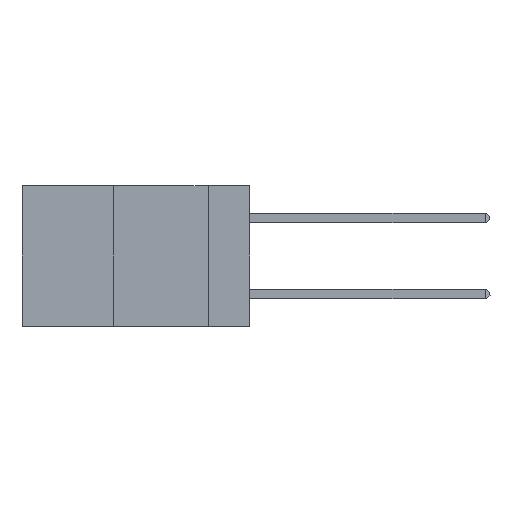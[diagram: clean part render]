
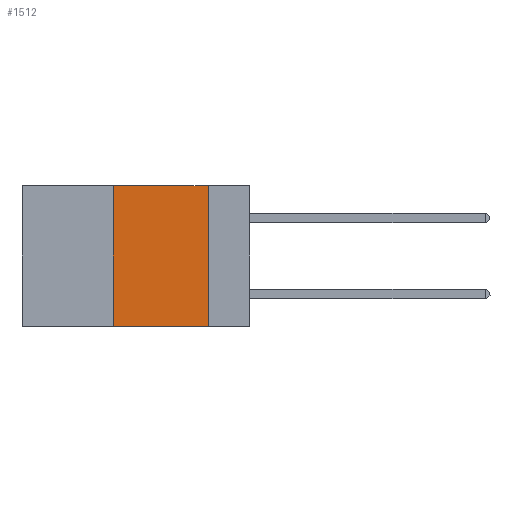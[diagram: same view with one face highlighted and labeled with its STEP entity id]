
A CAD part, left-side view. The second image highlights one B-rep face of the part: STEP entity #1512.
In plain terms, the highlighted planar face has unit normal (-1, 0, 0).
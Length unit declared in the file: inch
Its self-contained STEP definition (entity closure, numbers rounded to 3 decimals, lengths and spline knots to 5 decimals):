
#875 = VERTEX_POINT ( 'NONE', #9442 ) ;
#1187 = VECTOR ( 'NONE', #8809, 39.37008 ) ;
#1382 = PLANE ( 'NONE',  #9355 ) ;
#1512 = ADVANCED_FACE ( 'NONE', ( #8071 ), #1382, .F. ) ;
#1883 = VERTEX_POINT ( 'NONE', #3095 ) ;
#1942 = ORIENTED_EDGE ( 'NONE', *, *, #6858, .T. ) ;
#2199 = EDGE_LOOP ( 'NONE', ( #8537, #2297, #2607, #1942 ) ) ;
#2297 = ORIENTED_EDGE ( 'NONE', *, *, #10416, .F. ) ;
#2519 = CARTESIAN_POINT ( 'NONE',  ( 0., 0.11, 0. ) ) ;
#2555 = DIRECTION ( 'NONE',  ( 0., -1., 0. ) ) ;
#2586 = LINE ( 'NONE', #2689, #8052 ) ;
#2607 = ORIENTED_EDGE ( 'NONE', *, *, #7558, .F. ) ;
#2645 = CARTESIAN_POINT ( 'NONE',  ( 0., 0.11, 0. ) ) ;
#2689 = CARTESIAN_POINT ( 'NONE',  ( 0., 0.36, 0. ) ) ;
#3023 = DIRECTION ( 'NONE',  ( 0., 0., 1. ) ) ;
#3095 = CARTESIAN_POINT ( 'NONE',  ( 0., 0.36, 0. ) ) ;
#3147 = CARTESIAN_POINT ( 'NONE',  ( 0., 0.6, 0. ) ) ;
#4251 = VECTOR ( 'NONE', #7780, 39.37008 ) ;
#4694 = VECTOR ( 'NONE', #2555, 39.37008 ) ;
#5821 = DIRECTION ( 'NONE',  ( 0., 0., -1. ) ) ;
#5934 = DIRECTION ( 'NONE',  ( 1., 0., 0. ) ) ;
#6052 = VERTEX_POINT ( 'NONE', #2645 ) ;
#6630 = LINE ( 'NONE', #6940, #4251 ) ;
#6641 = LINE ( 'NONE', #8933, #4694 ) ;
#6803 = EDGE_CURVE ( 'NONE', #6052, #11433, #7208, .T. ) ;
#6858 = EDGE_CURVE ( 'NONE', #875, #11433, #6641, .T. ) ;
#6940 = CARTESIAN_POINT ( 'NONE',  ( 0., 0.6, 0. ) ) ;
#7208 = LINE ( 'NONE', #2519, #1187 ) ;
#7558 = EDGE_CURVE ( 'NONE', #875, #1883, #2586, .T. ) ;
#7780 = DIRECTION ( 'NONE',  ( 0., -1., 0. ) ) ;
#8052 = VECTOR ( 'NONE', #3023, 39.37008 ) ;
#8071 = FACE_OUTER_BOUND ( 'NONE', #2199, .T. ) ;
#8537 = ORIENTED_EDGE ( 'NONE', *, *, #6803, .F. ) ;
#8809 = DIRECTION ( 'NONE',  ( 0., 0., -1. ) ) ;
#8933 = CARTESIAN_POINT ( 'NONE',  ( 0., 0.6, -0.37 ) ) ;
#9355 = AXIS2_PLACEMENT_3D ( 'NONE', #3147, #5934, #5821 ) ;
#9441 = CARTESIAN_POINT ( 'NONE',  ( 0., 0.11, -0.37 ) ) ;
#9442 = CARTESIAN_POINT ( 'NONE',  ( 0., 0.36, -0.37 ) ) ;
#10416 = EDGE_CURVE ( 'NONE', #1883, #6052, #6630, .T. ) ;
#11433 = VERTEX_POINT ( 'NONE', #9441 ) ;
